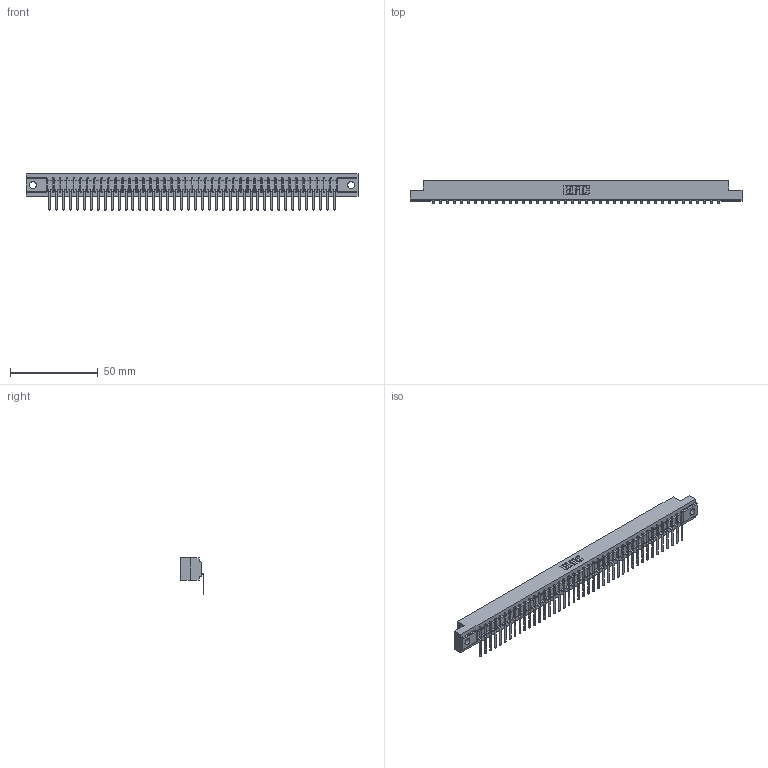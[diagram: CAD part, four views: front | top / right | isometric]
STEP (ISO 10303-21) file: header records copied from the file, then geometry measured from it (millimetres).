
FILE_DESCRIPTION (( 'STEP AP203' ), '1' );
FILE_NAME ('357-042-457-104.STEP', '2020-10-03T11:25:38', ( '' ), ( '' ), 'SwSTEP 2.0', 'SolidWorks 2020', '' );
FILE_SCHEMA (( 'CONFIG_CONTROL_DESIGN' ));
Length unit declared in the file: inch
Products named in the file (3): 307 Part_.156 Dia Mounting Holes; 357-042-457-104; 307-290-002_557
Assembly tree (43 placements, depth 2):
  357-042-457-104
    307 Part_.156 Dia Mounting Holes
    307-290-002_557  x42
Bounding box: 189.43 x 13.32 x 20.66 mm (x, y, z)
Volume: 20279.1 mm3; surface area: 26070.6 mm2
Topology: 43 solids, 43 shells, 3451 faces, 10607 edges, 6954 vertices
Faces by surface type: plane 2058, cylinder 1307, sphere 86
Entity records: 37278 total; most frequent: CARTESIAN_POINT 6294, ORIENTED_EDGE 6282, DIRECTION 6107, EDGE_CURVE 3141, LINE 2413, VECTOR 2413, VERTEX_POINT 2034, AXIS2_PLACEMENT_3D 1847
